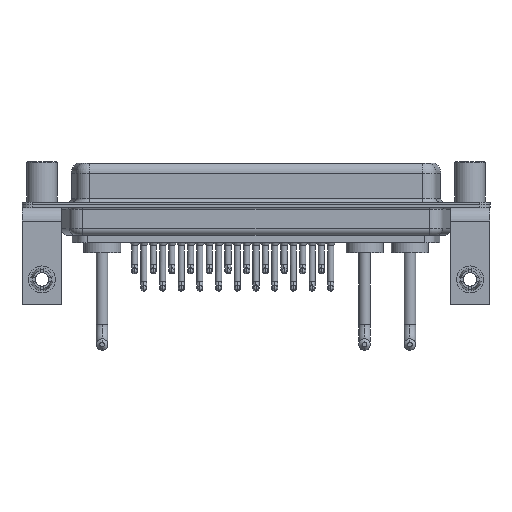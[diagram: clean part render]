
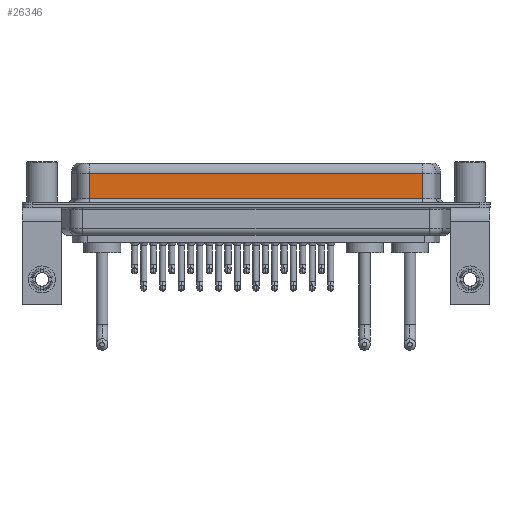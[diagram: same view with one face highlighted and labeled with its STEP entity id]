
A CAD part, front view. The second image highlights one B-rep face of the part: STEP entity #26346.
In plain terms, the highlighted planar face has unit normal (0, -1, 0).
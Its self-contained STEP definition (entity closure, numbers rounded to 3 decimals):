
#1771 = VECTOR ( 'NONE', #7736, 1000. ) ;
#1827 = CARTESIAN_POINT ( 'NONE',  ( 56.462, -3.95, 4.65 ) ) ;
#4077 = EDGE_CURVE ( 'NONE', #9607, #17382, #7438, .T. ) ;
#4831 = CARTESIAN_POINT ( 'NONE',  ( 56.462, -3.95, 6.4 ) ) ;
#5615 = AXIS2_PLACEMENT_3D ( 'NONE', #16873, #12568, #17146 ) ;
#6334 = CARTESIAN_POINT ( 'NONE',  ( 7.038, -3.95, 0.9 ) ) ;
#7438 = LINE ( 'NONE', #4831, #18488 ) ;
#7736 = DIRECTION ( 'NONE',  ( 0., 0., -1. ) ) ;
#8353 = CARTESIAN_POINT ( 'NONE',  ( 7.038, -3.95, 4.65 ) ) ;
#8560 = FACE_OUTER_BOUND ( 'NONE', #11446, .T. ) ;
#8615 = EDGE_CURVE ( 'NONE', #21250, #25101, #13974, .T. ) ;
#9174 = ORIENTED_EDGE ( 'NONE', *, *, #14945, .T. ) ;
#9607 = VERTEX_POINT ( 'NONE', #10418 ) ;
#9981 = ORIENTED_EDGE ( 'NONE', *, *, #4077, .F. ) ;
#9991 = LINE ( 'NONE', #1827, #21331 ) ;
#10418 = CARTESIAN_POINT ( 'NONE',  ( 56.462, -3.95, 4.65 ) ) ;
#11446 = EDGE_LOOP ( 'NONE', ( #9981, #24375, #11917, #9174 ) ) ;
#11917 = ORIENTED_EDGE ( 'NONE', *, *, #8615, .T. ) ;
#12107 = DIRECTION ( 'NONE',  ( 1., 0., 0. ) ) ;
#12568 = DIRECTION ( 'NONE',  ( 0., 1., 0. ) ) ;
#13974 = LINE ( 'NONE', #18255, #1771 ) ;
#14078 = VECTOR ( 'NONE', #12107, 1000. ) ;
#14945 = EDGE_CURVE ( 'NONE', #25101, #17382, #18752, .T. ) ;
#16556 = CARTESIAN_POINT ( 'NONE',  ( 56.462, -3.95, 0.9 ) ) ;
#16873 = CARTESIAN_POINT ( 'NONE',  ( 56.462, -3.95, 6.4 ) ) ;
#17146 = DIRECTION ( 'NONE',  ( 0., 0., 1. ) ) ;
#17382 = VERTEX_POINT ( 'NONE', #24001 ) ;
#18255 = CARTESIAN_POINT ( 'NONE',  ( 7.038, -3.95, 6.4 ) ) ;
#18488 = VECTOR ( 'NONE', #19492, 1000. ) ;
#18752 = LINE ( 'NONE', #16556, #14078 ) ;
#19492 = DIRECTION ( 'NONE',  ( 0., 0., -1. ) ) ;
#21250 = VERTEX_POINT ( 'NONE', #8353 ) ;
#21280 = PLANE ( 'NONE',  #5615 ) ;
#21331 = VECTOR ( 'NONE', #22867, 1000. ) ;
#22660 = EDGE_CURVE ( 'NONE', #9607, #21250, #9991, .T. ) ;
#22867 = DIRECTION ( 'NONE',  ( -1., 0., 0. ) ) ;
#24001 = CARTESIAN_POINT ( 'NONE',  ( 56.462, -3.95, 0.9 ) ) ;
#24375 = ORIENTED_EDGE ( 'NONE', *, *, #22660, .T. ) ;
#25101 = VERTEX_POINT ( 'NONE', #6334 ) ;
#26346 = ADVANCED_FACE ( 'NONE', ( #8560 ), #21280, .F. ) ;
